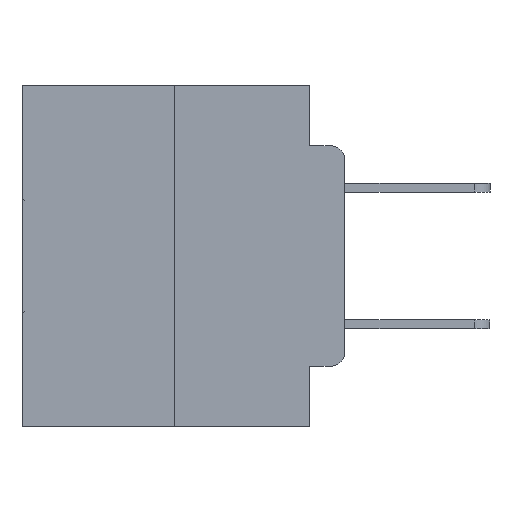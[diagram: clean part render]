
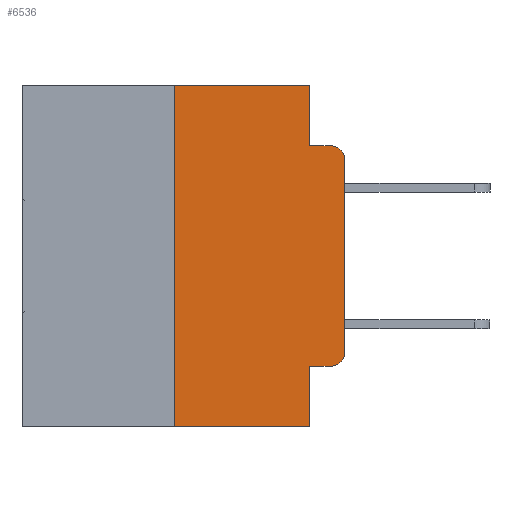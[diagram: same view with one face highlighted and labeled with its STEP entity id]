
A CAD part, left-side view. The second image highlights one B-rep face of the part: STEP entity #6536.
In plain terms, the highlighted planar face has unit normal (-1, 0, 0).
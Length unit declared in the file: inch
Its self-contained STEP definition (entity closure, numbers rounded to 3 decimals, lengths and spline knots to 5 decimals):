
#183 = CARTESIAN_POINT ( 'NONE',  ( 0., 0.473, -0.5 ) ) ;
#236 = AXIS2_PLACEMENT_3D ( 'NONE', #5139, #20835, #7390 ) ;
#476 = VERTEX_POINT ( 'NONE', #527 ) ;
#489 = LINE ( 'NONE', #16014, #11206 ) ;
#527 = CARTESIAN_POINT ( 'NONE',  ( 0., 0.051, -0.5 ) ) ;
#1006 = CARTESIAN_POINT ( 'NONE',  ( 0., 0.25, -0.5 ) ) ;
#2074 = EDGE_CURVE ( 'NONE', #23076, #15591, #22180, .T. ) ;
#2616 = DIRECTION ( 'NONE',  ( 0., -1., 0. ) ) ;
#3066 = LINE ( 'NONE', #16731, #19580 ) ;
#3453 = PLANE ( 'NONE',  #28467 ) ;
#3651 = EDGE_CURVE ( 'NONE', #18575, #23076, #489, .T. ) ;
#3968 = VERTEX_POINT ( 'NONE', #6001 ) ;
#4214 = EDGE_CURVE ( 'NONE', #25383, #14951, #3066, .T. ) ;
#5077 = CARTESIAN_POINT ( 'NONE',  ( 0., 0.02, -0.0885 ) ) ;
#5139 = CARTESIAN_POINT ( 'NONE',  ( 0., 0.02, -0.3915 ) ) ;
#5537 = CARTESIAN_POINT ( 'NONE',  ( 0., 0.02, -0.1085 ) ) ;
#5721 = DIRECTION ( 'NONE',  ( 1., 0., 0. ) ) ;
#6001 = CARTESIAN_POINT ( 'NONE',  ( 0., 0.25, 0. ) ) ;
#6285 = CARTESIAN_POINT ( 'NONE',  ( 0., 0.051, 0. ) ) ;
#6536 = ADVANCED_FACE ( 'NONE', ( #23470 ), #3453, .F. ) ;
#6768 = EDGE_CURVE ( 'NONE', #3968, #25383, #22407, .T. ) ;
#7058 = VECTOR ( 'NONE', #2616, 39.37008 ) ;
#7390 = DIRECTION ( 'NONE',  ( 0., 0., -1. ) ) ;
#7427 = ORIENTED_EDGE ( 'NONE', *, *, #3651, .T. ) ;
#7886 = CARTESIAN_POINT ( 'NONE',  ( 0., 0.473, 0. ) ) ;
#7999 = LINE ( 'NONE', #6285, #9404 ) ;
#8439 = ORIENTED_EDGE ( 'NONE', *, *, #4214, .F. ) ;
#8523 = DIRECTION ( 'NONE',  ( 0., 0., -1. ) ) ;
#8749 = DIRECTION ( 'NONE',  ( 0., -1., 0. ) ) ;
#9404 = VECTOR ( 'NONE', #8523, 39.37008 ) ;
#9935 = LINE ( 'NONE', #16816, #27827 ) ;
#10932 = CARTESIAN_POINT ( 'NONE',  ( 0., 0.051, -0.4115 ) ) ;
#11206 = VECTOR ( 'NONE', #14456, 39.37008 ) ;
#11269 = ORIENTED_EDGE ( 'NONE', *, *, #18317, .F. ) ;
#12360 = ORIENTED_EDGE ( 'NONE', *, *, #28250, .F. ) ;
#12609 = VERTEX_POINT ( 'NONE', #15291 ) ;
#12654 = VECTOR ( 'NONE', #13221, 39.37008 ) ;
#12829 = DIRECTION ( 'NONE',  ( 0., 0., -1. ) ) ;
#13039 = CARTESIAN_POINT ( 'NONE',  ( 0., 0.051, 0. ) ) ;
#13221 = DIRECTION ( 'NONE',  ( 0., -1., 0. ) ) ;
#13785 = CARTESIAN_POINT ( 'NONE',  ( 0., 0., -0.1085 ) ) ;
#13954 = CARTESIAN_POINT ( 'NONE',  ( 0., 0.051, -0.0885 ) ) ;
#14456 = DIRECTION ( 'NONE',  ( 0., 0., 1. ) ) ;
#14951 = VERTEX_POINT ( 'NONE', #13954 ) ;
#15291 = CARTESIAN_POINT ( 'NONE',  ( 0., 0.051, -0.4115 ) ) ;
#15591 = VERTEX_POINT ( 'NONE', #5077 ) ;
#16014 = CARTESIAN_POINT ( 'NONE',  ( 0., 0., 0. ) ) ;
#16168 = ORIENTED_EDGE ( 'NONE', *, *, #2074, .T. ) ;
#16423 = VECTOR ( 'NONE', #8749, 39.37008 ) ;
#16731 = CARTESIAN_POINT ( 'NONE',  ( 0., 0.051, 0. ) ) ;
#16816 = CARTESIAN_POINT ( 'NONE',  ( 0., 0.25, 0. ) ) ;
#16825 = ORIENTED_EDGE ( 'NONE', *, *, #6768, .F. ) ;
#16944 = VERTEX_POINT ( 'NONE', #1006 ) ;
#17121 = ORIENTED_EDGE ( 'NONE', *, *, #25825, .F. ) ;
#17873 = AXIS2_PLACEMENT_3D ( 'NONE', #5537, #19322, #24482 ) ;
#18003 = CARTESIAN_POINT ( 'NONE',  ( 0., 0.051, -0.0885 ) ) ;
#18273 = LINE ( 'NONE', #183, #7058 ) ;
#18317 = EDGE_CURVE ( 'NONE', #12609, #476, #7999, .T. ) ;
#18575 = VERTEX_POINT ( 'NONE', #27337 ) ;
#18930 = ORIENTED_EDGE ( 'NONE', *, *, #23106, .T. ) ;
#19073 = DIRECTION ( 'NONE',  ( 0., 0., 1. ) ) ;
#19322 = DIRECTION ( 'NONE',  ( -1., 0., 0. ) ) ;
#19580 = VECTOR ( 'NONE', #12829, 39.37008 ) ;
#20153 = ORIENTED_EDGE ( 'NONE', *, *, #24892, .T. ) ;
#20303 = DIRECTION ( 'NONE',  ( 0., -1., 0. ) ) ;
#20706 = VECTOR ( 'NONE', #20303, 39.37008 ) ;
#20835 = DIRECTION ( 'NONE',  ( -1., 0., 0. ) ) ;
#21437 = DIRECTION ( 'NONE',  ( 0., 0., -1. ) ) ;
#22180 = CIRCLE ( 'NONE', #17873, 0.02 ) ;
#22407 = LINE ( 'NONE', #24438, #16423 ) ;
#22455 = VERTEX_POINT ( 'NONE', #22722 ) ;
#22722 = CARTESIAN_POINT ( 'NONE',  ( 0., 0.02, -0.4115 ) ) ;
#23076 = VERTEX_POINT ( 'NONE', #13785 ) ;
#23106 = EDGE_CURVE ( 'NONE', #16944, #476, #18273, .T. ) ;
#23470 = FACE_OUTER_BOUND ( 'NONE', #23974, .T. ) ;
#23974 = EDGE_LOOP ( 'NONE', ( #7427, #16168, #12360, #8439, #16825, #17121, #18930, #11269, #28202, #20153 ) ) ;
#24438 = CARTESIAN_POINT ( 'NONE',  ( 0., 0.473, 0. ) ) ;
#24482 = DIRECTION ( 'NONE',  ( 0., 0., -1. ) ) ;
#24892 = EDGE_CURVE ( 'NONE', #22455, #18575, #28182, .T. ) ;
#25267 = LINE ( 'NONE', #10932, #12654 ) ;
#25383 = VERTEX_POINT ( 'NONE', #13039 ) ;
#25825 = EDGE_CURVE ( 'NONE', #16944, #3968, #9935, .T. ) ;
#27332 = LINE ( 'NONE', #18003, #20706 ) ;
#27337 = CARTESIAN_POINT ( 'NONE',  ( 0., 0., -0.3915 ) ) ;
#27827 = VECTOR ( 'NONE', #19073, 39.37008 ) ;
#27882 = EDGE_CURVE ( 'NONE', #12609, #22455, #25267, .T. ) ;
#28182 = CIRCLE ( 'NONE', #236, 0.02 ) ;
#28202 = ORIENTED_EDGE ( 'NONE', *, *, #27882, .T. ) ;
#28250 = EDGE_CURVE ( 'NONE', #14951, #15591, #27332, .T. ) ;
#28467 = AXIS2_PLACEMENT_3D ( 'NONE', #7886, #5721, #21437 ) ;
